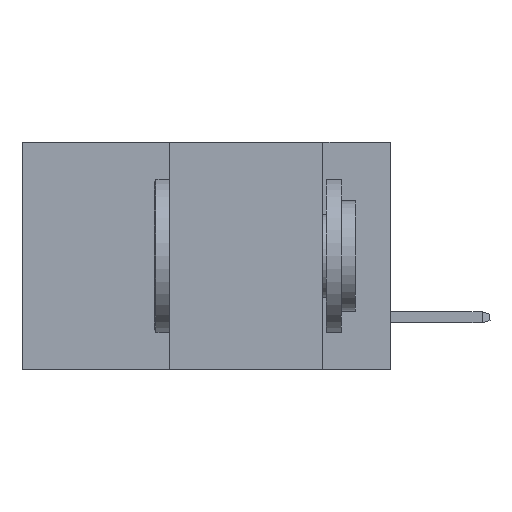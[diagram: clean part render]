
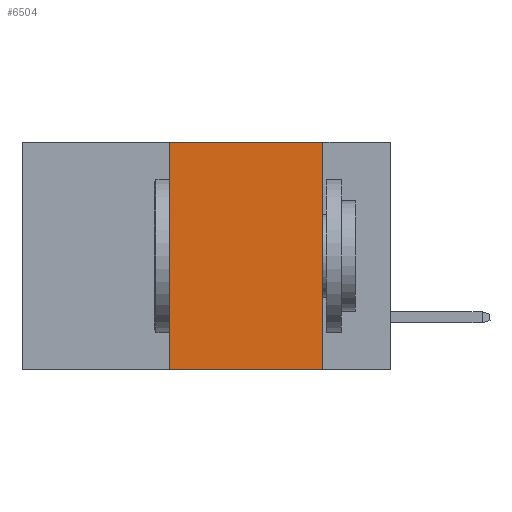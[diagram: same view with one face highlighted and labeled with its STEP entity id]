
A CAD part, left-side view. The second image highlights one B-rep face of the part: STEP entity #6504.
In plain terms, the highlighted planar face has unit normal (-1, 0, 0).
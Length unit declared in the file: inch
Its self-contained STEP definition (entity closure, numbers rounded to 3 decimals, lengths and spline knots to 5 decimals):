
#351 = ORIENTED_EDGE ( 'NONE', *, *, #6776, .F. ) ;
#611 = AXIS2_PLACEMENT_3D ( 'NONE', #1663, #5116, #8326 ) ;
#913 = DIRECTION ( 'NONE',  ( 0., -1., 0. ) ) ;
#1556 = EDGE_CURVE ( 'NONE', #14470, #8865, #5172, .T. ) ;
#1663 = CARTESIAN_POINT ( 'NONE',  ( 0., 0.6, 0. ) ) ;
#1836 = CARTESIAN_POINT ( 'NONE',  ( 0., 0.6, 0. ) ) ;
#3190 = EDGE_CURVE ( 'NONE', #13952, #5308, #14468, .T. ) ;
#4406 = VECTOR ( 'NONE', #6341, 39.37008 ) ;
#4465 = VECTOR ( 'NONE', #13182, 39.37008 ) ;
#4752 = CARTESIAN_POINT ( 'NONE',  ( 0., 0.36, 0. ) ) ;
#4849 = VECTOR ( 'NONE', #11847, 39.37008 ) ;
#5116 = DIRECTION ( 'NONE',  ( 1., 0., 0. ) ) ;
#5172 = LINE ( 'NONE', #1836, #4465 ) ;
#5308 = VERTEX_POINT ( 'NONE', #11756 ) ;
#5749 = ORIENTED_EDGE ( 'NONE', *, *, #3190, .T. ) ;
#6341 = DIRECTION ( 'NONE',  ( 0., 0., -1. ) ) ;
#6349 = FACE_OUTER_BOUND ( 'NONE', #6892, .T. ) ;
#6504 = ADVANCED_FACE ( 'NONE', ( #6349 ), #10755, .F. ) ;
#6776 = EDGE_CURVE ( 'NONE', #8865, #5308, #13218, .T. ) ;
#6892 = EDGE_LOOP ( 'NONE', ( #351, #7016, #11066, #5749 ) ) ;
#7016 = ORIENTED_EDGE ( 'NONE', *, *, #1556, .F. ) ;
#7593 = CARTESIAN_POINT ( 'NONE',  ( 0., 0.6, -0.37 ) ) ;
#8196 = LINE ( 'NONE', #4752, #4849 ) ;
#8326 = DIRECTION ( 'NONE',  ( 0., 0., -1. ) ) ;
#8372 = CARTESIAN_POINT ( 'NONE',  ( 0., 0.11, 0. ) ) ;
#8865 = VERTEX_POINT ( 'NONE', #8372 ) ;
#10755 = PLANE ( 'NONE',  #611 ) ;
#11066 = ORIENTED_EDGE ( 'NONE', *, *, #13725, .F. ) ;
#11104 = CARTESIAN_POINT ( 'NONE',  ( 0., 0.36, 0. ) ) ;
#11489 = VECTOR ( 'NONE', #913, 39.37008 ) ;
#11756 = CARTESIAN_POINT ( 'NONE',  ( 0., 0.11, -0.37 ) ) ;
#11847 = DIRECTION ( 'NONE',  ( 0., 0., 1. ) ) ;
#12762 = CARTESIAN_POINT ( 'NONE',  ( 0., 0.36, -0.37 ) ) ;
#13182 = DIRECTION ( 'NONE',  ( 0., -1., 0. ) ) ;
#13205 = CARTESIAN_POINT ( 'NONE',  ( 0., 0.11, 0. ) ) ;
#13218 = LINE ( 'NONE', #13205, #4406 ) ;
#13725 = EDGE_CURVE ( 'NONE', #13952, #14470, #8196, .T. ) ;
#13952 = VERTEX_POINT ( 'NONE', #12762 ) ;
#14468 = LINE ( 'NONE', #7593, #11489 ) ;
#14470 = VERTEX_POINT ( 'NONE', #11104 ) ;
